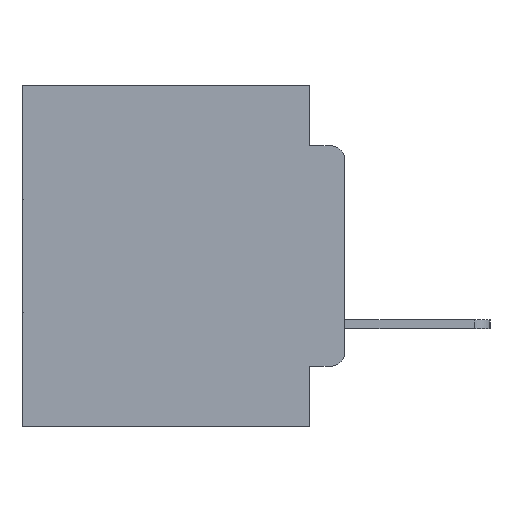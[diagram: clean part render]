
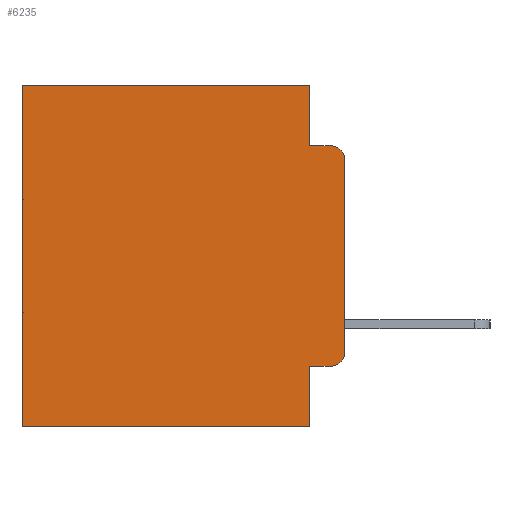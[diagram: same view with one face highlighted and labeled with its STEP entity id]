
A CAD part, left-side view. The second image highlights one B-rep face of the part: STEP entity #6235.
In plain terms, the highlighted planar face has unit normal (-1, 0, 0).
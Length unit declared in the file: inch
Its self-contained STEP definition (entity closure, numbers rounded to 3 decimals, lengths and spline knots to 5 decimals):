
#3 = CARTESIAN_POINT ( 'NONE',  ( 0.298, 0.02, -0.1085 ) ) ;
#572 = DIRECTION ( 'NONE',  ( 0., 0., -1. ) ) ;
#1520 = EDGE_CURVE ( 'NONE', #27200, #25387, #1601, .T. ) ;
#1601 = LINE ( 'NONE', #21502, #12216 ) ;
#2455 = VERTEX_POINT ( 'NONE', #7050 ) ;
#3111 = EDGE_CURVE ( 'NONE', #19041, #25387, #8670, .T. ) ;
#3208 = DIRECTION ( 'NONE',  ( 0., -1., 0. ) ) ;
#4025 = DIRECTION ( 'NONE',  ( 0., 0., -1. ) ) ;
#4048 = DIRECTION ( 'NONE',  ( 0., 1., 0. ) ) ;
#4121 = VERTEX_POINT ( 'NONE', #4810 ) ;
#4268 = AXIS2_PLACEMENT_3D ( 'NONE', #6282, #17424, #4025 ) ;
#4779 = ORIENTED_EDGE ( 'NONE', *, *, #1520, .F. ) ;
#4810 = CARTESIAN_POINT ( 'NONE',  ( 0.298, 0.473, 0. ) ) ;
#5150 = VERTEX_POINT ( 'NONE', #12198 ) ;
#5220 = VERTEX_POINT ( 'NONE', #25974 ) ;
#5236 = LINE ( 'NONE', #28169, #28663 ) ;
#5545 = CARTESIAN_POINT ( 'NONE',  ( 0.298, 0.051, 0. ) ) ;
#5617 = VECTOR ( 'NONE', #16678, 39.37008 ) ;
#5886 = ORIENTED_EDGE ( 'NONE', *, *, #22973, .T. ) ;
#5922 = AXIS2_PLACEMENT_3D ( 'NONE', #3, #9757, #18421 ) ;
#6235 = ADVANCED_FACE ( 'NONE', ( #8876 ), #15741, .F. ) ;
#6282 = CARTESIAN_POINT ( 'NONE',  ( 0.298, 0., 0. ) ) ;
#6932 = EDGE_CURVE ( 'NONE', #20897, #7964, #8474, .T. ) ;
#7050 = CARTESIAN_POINT ( 'NONE',  ( 0.298, 0.051, -0.4115 ) ) ;
#7172 = CARTESIAN_POINT ( 'NONE',  ( 0.298, 0.02, -0.4115 ) ) ;
#7964 = VERTEX_POINT ( 'NONE', #15711 ) ;
#8096 = CARTESIAN_POINT ( 'NONE',  ( 0.298, 0.051, -0.0885 ) ) ;
#8474 = LINE ( 'NONE', #19785, #20229 ) ;
#8670 = CIRCLE ( 'NONE', #5922, 0.02 ) ;
#8876 = FACE_OUTER_BOUND ( 'NONE', #18663, .T. ) ;
#9409 = CARTESIAN_POINT ( 'NONE',  ( 0.298, 0.051, -0.4115 ) ) ;
#9757 = DIRECTION ( 'NONE',  ( -1., 0., 0. ) ) ;
#10459 = ORIENTED_EDGE ( 'NONE', *, *, #6932, .F. ) ;
#10833 = VECTOR ( 'NONE', #26012, 39.37008 ) ;
#11466 = ORIENTED_EDGE ( 'NONE', *, *, #13626, .F. ) ;
#11567 = LINE ( 'NONE', #5545, #5617 ) ;
#11770 = LINE ( 'NONE', #24976, #28543 ) ;
#11827 = ORIENTED_EDGE ( 'NONE', *, *, #18658, .T. ) ;
#12198 = CARTESIAN_POINT ( 'NONE',  ( 0.298, 0., -0.3915 ) ) ;
#12216 = VECTOR ( 'NONE', #3208, 39.37008 ) ;
#12690 = EDGE_CURVE ( 'NONE', #27559, #5150, #26336, .T. ) ;
#12857 = CARTESIAN_POINT ( 'NONE',  ( 0.298, 0., -0.1085 ) ) ;
#13626 = EDGE_CURVE ( 'NONE', #19041, #5150, #5236, .T. ) ;
#14163 = DIRECTION ( 'NONE',  ( -1., 0., 0. ) ) ;
#14561 = ORIENTED_EDGE ( 'NONE', *, *, #28826, .F. ) ;
#15207 = LINE ( 'NONE', #26064, #25436 ) ;
#15711 = CARTESIAN_POINT ( 'NONE',  ( 0.298, 0.473, -0.5 ) ) ;
#15741 = PLANE ( 'NONE',  #4268 ) ;
#16578 = EDGE_CURVE ( 'NONE', #5220, #4121, #15207, .T. ) ;
#16678 = DIRECTION ( 'NONE',  ( 0., 0., -1. ) ) ;
#17346 = DIRECTION ( 'NONE',  ( 0., 0., -1. ) ) ;
#17424 = DIRECTION ( 'NONE',  ( 1., 0., 0. ) ) ;
#18421 = DIRECTION ( 'NONE',  ( 0., 0., -1. ) ) ;
#18470 = DIRECTION ( 'NONE',  ( 0., 0., -1. ) ) ;
#18658 = EDGE_CURVE ( 'NONE', #2455, #27559, #22916, .T. ) ;
#18663 = EDGE_LOOP ( 'NONE', ( #11466, #26858, #4779, #14561, #21098, #5886, #10459, #23473, #11827, #24854 ) ) ;
#19041 = VERTEX_POINT ( 'NONE', #12857 ) ;
#19785 = CARTESIAN_POINT ( 'NONE',  ( 0.298, 0., -0.5 ) ) ;
#20229 = VECTOR ( 'NONE', #22074, 39.37008 ) ;
#20897 = VERTEX_POINT ( 'NONE', #26262 ) ;
#21098 = ORIENTED_EDGE ( 'NONE', *, *, #16578, .T. ) ;
#21502 = CARTESIAN_POINT ( 'NONE',  ( 0.298, 0.051, -0.0885 ) ) ;
#21554 = EDGE_CURVE ( 'NONE', #2455, #20897, #28304, .T. ) ;
#22074 = DIRECTION ( 'NONE',  ( 0., 1., 0. ) ) ;
#22558 = DIRECTION ( 'NONE',  ( 0., -1., 0. ) ) ;
#22916 = LINE ( 'NONE', #9409, #27355 ) ;
#22973 = EDGE_CURVE ( 'NONE', #4121, #7964, #11770, .T. ) ;
#23473 = ORIENTED_EDGE ( 'NONE', *, *, #21554, .F. ) ;
#23810 = CARTESIAN_POINT ( 'NONE',  ( 0.298, 0.02, -0.0885 ) ) ;
#24854 = ORIENTED_EDGE ( 'NONE', *, *, #12690, .T. ) ;
#24976 = CARTESIAN_POINT ( 'NONE',  ( 0.298, 0.473, 0. ) ) ;
#25387 = VERTEX_POINT ( 'NONE', #23810 ) ;
#25436 = VECTOR ( 'NONE', #4048, 39.37008 ) ;
#25974 = CARTESIAN_POINT ( 'NONE',  ( 0.298, 0.051, 0. ) ) ;
#26012 = DIRECTION ( 'NONE',  ( 0., 0., -1. ) ) ;
#26064 = CARTESIAN_POINT ( 'NONE',  ( 0.298, 0., 0. ) ) ;
#26262 = CARTESIAN_POINT ( 'NONE',  ( 0.298, 0.051, -0.5 ) ) ;
#26336 = CIRCLE ( 'NONE', #27738, 0.02 ) ;
#26858 = ORIENTED_EDGE ( 'NONE', *, *, #3111, .T. ) ;
#27200 = VERTEX_POINT ( 'NONE', #8096 ) ;
#27252 = CARTESIAN_POINT ( 'NONE',  ( 0.298, 0.02, -0.3915 ) ) ;
#27355 = VECTOR ( 'NONE', #22558, 39.37008 ) ;
#27559 = VERTEX_POINT ( 'NONE', #7172 ) ;
#27738 = AXIS2_PLACEMENT_3D ( 'NONE', #27252, #14163, #572 ) ;
#28169 = CARTESIAN_POINT ( 'NONE',  ( 0.298, 0., 0. ) ) ;
#28219 = CARTESIAN_POINT ( 'NONE',  ( 0.298, 0.051, 0. ) ) ;
#28304 = LINE ( 'NONE', #28219, #10833 ) ;
#28543 = VECTOR ( 'NONE', #18470, 39.37008 ) ;
#28663 = VECTOR ( 'NONE', #17346, 39.37008 ) ;
#28826 = EDGE_CURVE ( 'NONE', #5220, #27200, #11567, .T. ) ;
